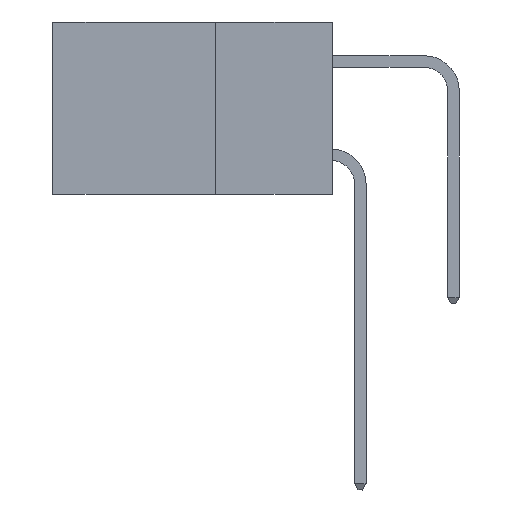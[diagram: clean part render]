
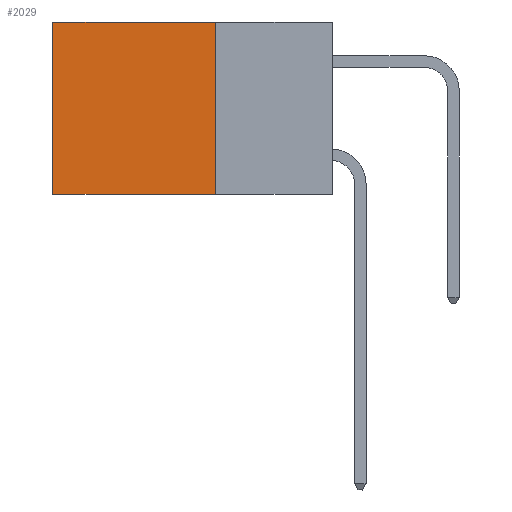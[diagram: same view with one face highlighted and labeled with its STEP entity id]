
A CAD part, left-side view. The second image highlights one B-rep face of the part: STEP entity #2029.
In plain terms, the highlighted planar face has unit normal (-1, 0, 0).
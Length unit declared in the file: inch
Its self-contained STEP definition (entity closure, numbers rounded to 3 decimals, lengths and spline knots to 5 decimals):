
#44 = ORIENTED_EDGE ( 'NONE', *, *, #12300, .F. ) ;
#2029 = ADVANCED_FACE ( 'NONE', ( #8932 ), #17466, .F. ) ;
#3300 = CARTESIAN_POINT ( 'NONE',  ( 0.2615, 0.6, -0.37 ) ) ;
#3524 = LINE ( 'NONE', #5585, #26442 ) ;
#4008 = EDGE_CURVE ( 'NONE', #25629, #4400, #22202, .T. ) ;
#4147 = CARTESIAN_POINT ( 'NONE',  ( 0.2615, 0.25, -0.37 ) ) ;
#4302 = LINE ( 'NONE', #16568, #25274 ) ;
#4400 = VERTEX_POINT ( 'NONE', #18095 ) ;
#5213 = DIRECTION ( 'NONE',  ( 0., 0., -1. ) ) ;
#5585 = CARTESIAN_POINT ( 'NONE',  ( 0.2615, 0.25, -0.37 ) ) ;
#6894 = VECTOR ( 'NONE', #11682, 39.37008 ) ;
#6992 = CARTESIAN_POINT ( 'NONE',  ( 0.2615, 0.25, -0.37 ) ) ;
#8838 = VERTEX_POINT ( 'NONE', #21840 ) ;
#8932 = FACE_OUTER_BOUND ( 'NONE', #18250, .T. ) ;
#9230 = LINE ( 'NONE', #26239, #24295 ) ;
#9333 = DIRECTION ( 'NONE',  ( 1., 0., 0. ) ) ;
#9431 = AXIS2_PLACEMENT_3D ( 'NONE', #6992, #9333, #25800 ) ;
#10922 = DIRECTION ( 'NONE',  ( 0., 1., 0. ) ) ;
#11009 = ORIENTED_EDGE ( 'NONE', *, *, #4008, .T. ) ;
#11507 = DIRECTION ( 'NONE',  ( 0., 1., 0. ) ) ;
#11682 = DIRECTION ( 'NONE',  ( 0., 0., -1. ) ) ;
#12300 = EDGE_CURVE ( 'NONE', #21544, #4400, #3524, .T. ) ;
#13132 = ORIENTED_EDGE ( 'NONE', *, *, #23425, .F. ) ;
#16568 = CARTESIAN_POINT ( 'NONE',  ( 0.2615, 0.25, 0. ) ) ;
#17080 = ORIENTED_EDGE ( 'NONE', *, *, #19365, .T. ) ;
#17280 = CARTESIAN_POINT ( 'NONE',  ( 0.2615, 0.6, 0. ) ) ;
#17466 = PLANE ( 'NONE',  #9431 ) ;
#18095 = CARTESIAN_POINT ( 'NONE',  ( 0.2615, 0.6, -0.37 ) ) ;
#18250 = EDGE_LOOP ( 'NONE', ( #11009, #44, #13132, #17080 ) ) ;
#19365 = EDGE_CURVE ( 'NONE', #8838, #25629, #4302, .T. ) ;
#21544 = VERTEX_POINT ( 'NONE', #4147 ) ;
#21840 = CARTESIAN_POINT ( 'NONE',  ( 0.2615, 0.25, 0. ) ) ;
#22202 = LINE ( 'NONE', #3300, #6894 ) ;
#23425 = EDGE_CURVE ( 'NONE', #8838, #21544, #9230, .T. ) ;
#24295 = VECTOR ( 'NONE', #5213, 39.37008 ) ;
#25274 = VECTOR ( 'NONE', #10922, 39.37008 ) ;
#25629 = VERTEX_POINT ( 'NONE', #17280 ) ;
#25800 = DIRECTION ( 'NONE',  ( 0., 0., -1. ) ) ;
#26239 = CARTESIAN_POINT ( 'NONE',  ( 0.2615, 0.25, -0.37 ) ) ;
#26442 = VECTOR ( 'NONE', #11507, 39.37008 ) ;
